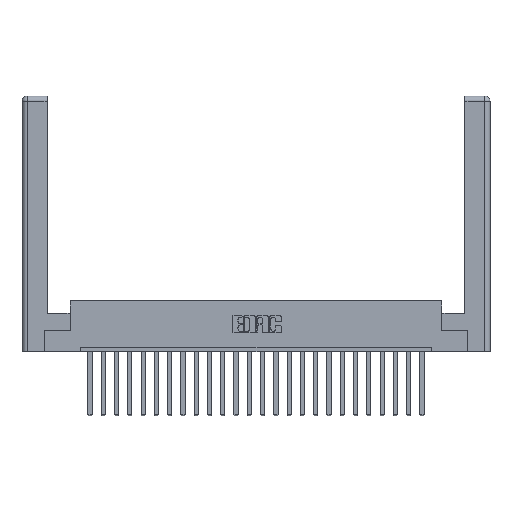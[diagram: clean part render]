
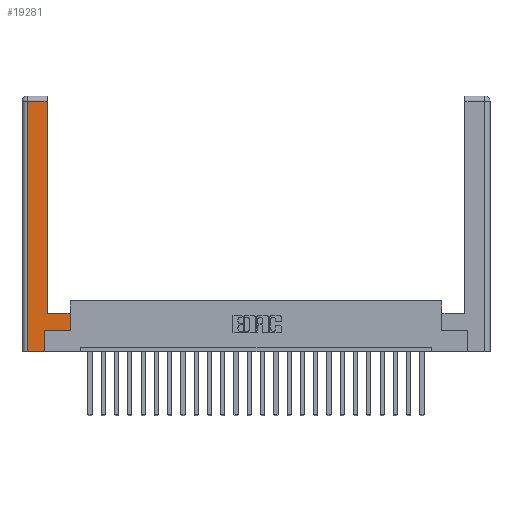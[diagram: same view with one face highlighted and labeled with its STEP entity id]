
A CAD part, top view. The second image highlights one B-rep face of the part: STEP entity #19281.
In plain terms, the highlighted planar face has unit normal (0, 0, 1).
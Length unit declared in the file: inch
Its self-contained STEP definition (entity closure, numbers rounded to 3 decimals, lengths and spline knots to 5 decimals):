
#28 = ORIENTED_EDGE ( 'NONE', *, *, #1547, .T. ) ;
#828 = CARTESIAN_POINT ( 'NONE',  ( 0.295, 2.94, 0. ) ) ;
#1034 = VERTEX_POINT ( 'NONE', #10036 ) ;
#1547 = EDGE_CURVE ( 'NONE', #17965, #17053, #23699, .T. ) ;
#2122 = VECTOR ( 'NONE', #22277, 39.37008 ) ;
#2752 = DIRECTION ( 'NONE',  ( 0., 1., 0. ) ) ;
#3330 = AXIS2_PLACEMENT_3D ( 'NONE', #19092, #11551, #13419 ) ;
#3495 = VERTEX_POINT ( 'NONE', #3557 ) ;
#3557 = CARTESIAN_POINT ( 'NONE',  ( 0.0615, 2.94, 0. ) ) ;
#3591 = LINE ( 'NONE', #4489, #10261 ) ;
#4489 = CARTESIAN_POINT ( 'NONE',  ( 0.565, 0.45, 0. ) ) ;
#4549 = CARTESIAN_POINT ( 'NONE',  ( 0.265, 0.245, 0. ) ) ;
#4599 = CARTESIAN_POINT ( 'NONE',  ( 0.295, 0.45, 0. ) ) ;
#4706 = CARTESIAN_POINT ( 'NONE',  ( 0.565, 0.245, 0. ) ) ;
#4792 = DIRECTION ( 'NONE',  ( 1., 0., 0. ) ) ;
#5373 = EDGE_CURVE ( 'NONE', #3495, #19639, #22560, .T. ) ;
#6993 = EDGE_CURVE ( 'NONE', #8597, #12825, #16251, .T. ) ;
#7816 = ORIENTED_EDGE ( 'NONE', *, *, #5373, .T. ) ;
#8597 = VERTEX_POINT ( 'NONE', #9299 ) ;
#8922 = CARTESIAN_POINT ( 'NONE',  ( 0.295, 0.45, 0. ) ) ;
#9299 = CARTESIAN_POINT ( 'NONE',  ( 0.565, 0.45, 0. ) ) ;
#9812 = DIRECTION ( 'NONE',  ( -1., 0., 0. ) ) ;
#10036 = CARTESIAN_POINT ( 'NONE',  ( 0.565, 0.245, 0. ) ) ;
#10064 = ORIENTED_EDGE ( 'NONE', *, *, #19006, .T. ) ;
#10261 = VECTOR ( 'NONE', #13626, 39.37008 ) ;
#10675 = VECTOR ( 'NONE', #17572, 39.37008 ) ;
#11551 = DIRECTION ( 'NONE',  ( 0., 0., -1. ) ) ;
#11845 = LINE ( 'NONE', #4706, #10675 ) ;
#12125 = CARTESIAN_POINT ( 'NONE',  ( 0.265, 0., 0. ) ) ;
#12411 = ORIENTED_EDGE ( 'NONE', *, *, #23470, .T. ) ;
#12477 = EDGE_CURVE ( 'NONE', #12825, #12499, #12598, .T. ) ;
#12499 = VERTEX_POINT ( 'NONE', #828 ) ;
#12598 = LINE ( 'NONE', #22936, #19484 ) ;
#12825 = VERTEX_POINT ( 'NONE', #8922 ) ;
#12981 = CARTESIAN_POINT ( 'NONE',  ( 0.265, 0., 0. ) ) ;
#13419 = DIRECTION ( 'NONE',  ( -1., 0., 0. ) ) ;
#13626 = DIRECTION ( 'NONE',  ( 0., 1., 0. ) ) ;
#13750 = EDGE_LOOP ( 'NONE', ( #17613, #21213, #7816, #15638, #28, #12411, #10064, #18317 ) ) ;
#14128 = EDGE_CURVE ( 'NONE', #19639, #17965, #22007, .T. ) ;
#14564 = VECTOR ( 'NONE', #4792, 39.37008 ) ;
#14711 = CARTESIAN_POINT ( 'NONE',  ( 0.0615, 0., 0. ) ) ;
#15418 = PLANE ( 'NONE',  #3330 ) ;
#15610 = CARTESIAN_POINT ( 'NONE',  ( 0.0615, 2.94, 0. ) ) ;
#15638 = ORIENTED_EDGE ( 'NONE', *, *, #14128, .T. ) ;
#16251 = LINE ( 'NONE', #4599, #19393 ) ;
#17053 = VERTEX_POINT ( 'NONE', #4549 ) ;
#17151 = DIRECTION ( 'NONE',  ( -1., 0., 0. ) ) ;
#17572 = DIRECTION ( 'NONE',  ( 1., 0., 0. ) ) ;
#17613 = ORIENTED_EDGE ( 'NONE', *, *, #12477, .T. ) ;
#17965 = VERTEX_POINT ( 'NONE', #12981 ) ;
#17968 = VECTOR ( 'NONE', #20392, 39.37008 ) ;
#18192 = CARTESIAN_POINT ( 'NONE',  ( 0.0615, 0., 0. ) ) ;
#18317 = ORIENTED_EDGE ( 'NONE', *, *, #6993, .T. ) ;
#19006 = EDGE_CURVE ( 'NONE', #1034, #8597, #3591, .T. ) ;
#19092 = CARTESIAN_POINT ( 'NONE',  ( 0., 0., 0. ) ) ;
#19281 = ADVANCED_FACE ( 'NONE', ( #21112 ), #15418, .F. ) ;
#19393 = VECTOR ( 'NONE', #17151, 39.37008 ) ;
#19484 = VECTOR ( 'NONE', #2752, 39.37008 ) ;
#19639 = VERTEX_POINT ( 'NONE', #18192 ) ;
#20392 = DIRECTION ( 'NONE',  ( 0., -1., 0. ) ) ;
#21112 = FACE_OUTER_BOUND ( 'NONE', #13750, .T. ) ;
#21213 = ORIENTED_EDGE ( 'NONE', *, *, #22886, .T. ) ;
#21643 = VECTOR ( 'NONE', #9812, 39.37008 ) ;
#22007 = LINE ( 'NONE', #12125, #14564 ) ;
#22114 = CARTESIAN_POINT ( 'NONE',  ( 0.265, 0.245, 0. ) ) ;
#22200 = LINE ( 'NONE', #15610, #21643 ) ;
#22277 = DIRECTION ( 'NONE',  ( 0., 1., 0. ) ) ;
#22560 = LINE ( 'NONE', #14711, #17968 ) ;
#22886 = EDGE_CURVE ( 'NONE', #12499, #3495, #22200, .T. ) ;
#22936 = CARTESIAN_POINT ( 'NONE',  ( 0.295, 3., 0. ) ) ;
#23470 = EDGE_CURVE ( 'NONE', #17053, #1034, #11845, .T. ) ;
#23699 = LINE ( 'NONE', #22114, #2122 ) ;
